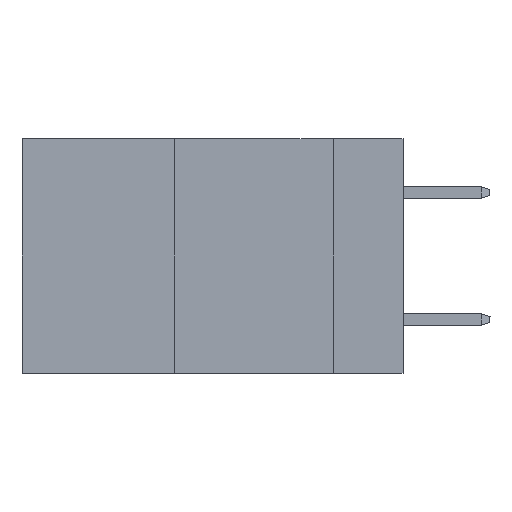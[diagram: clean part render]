
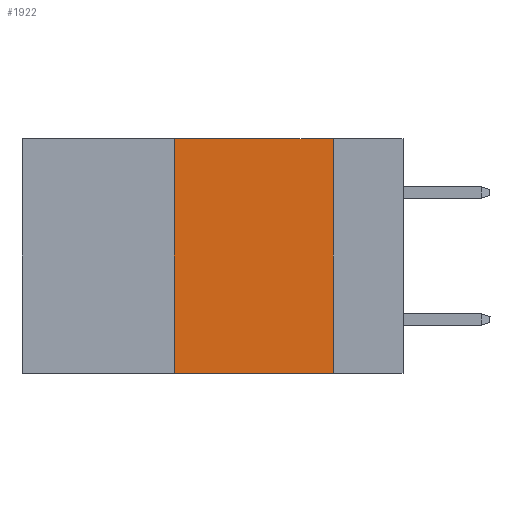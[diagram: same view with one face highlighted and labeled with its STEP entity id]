
A CAD part, left-side view. The second image highlights one B-rep face of the part: STEP entity #1922.
In plain terms, the highlighted planar face has unit normal (-1, 0, 0).
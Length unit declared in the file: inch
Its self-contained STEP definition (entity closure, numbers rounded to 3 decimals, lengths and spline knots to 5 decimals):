
#661 = CARTESIAN_POINT ( 'NONE',  ( 0., 0.11, -0.37 ) ) ;
#853 = ORIENTED_EDGE ( 'NONE', *, *, #22373, .F. ) ;
#1360 = VECTOR ( 'NONE', #24112, 39.37008 ) ;
#1922 = ADVANCED_FACE ( 'NONE', ( #19017 ), #7558, .F. ) ;
#2053 = EDGE_CURVE ( 'NONE', #28522, #11244, #5907, .T. ) ;
#2545 = LINE ( 'NONE', #27266, #9186 ) ;
#3667 = CARTESIAN_POINT ( 'NONE',  ( 0., 0.36, -0.37 ) ) ;
#5485 = LINE ( 'NONE', #28543, #5537 ) ;
#5537 = VECTOR ( 'NONE', #14390, 39.37008 ) ;
#5697 = CARTESIAN_POINT ( 'NONE',  ( 0., 0.6, -0.37 ) ) ;
#5907 = LINE ( 'NONE', #10567, #8036 ) ;
#6410 = VERTEX_POINT ( 'NONE', #3667 ) ;
#6632 = AXIS2_PLACEMENT_3D ( 'NONE', #14051, #23275, #7260 ) ;
#7260 = DIRECTION ( 'NONE',  ( 0., 0., -1. ) ) ;
#7558 = PLANE ( 'NONE',  #6632 ) ;
#8036 = VECTOR ( 'NONE', #24327, 39.37008 ) ;
#8300 = CARTESIAN_POINT ( 'NONE',  ( 0., 0.11, 0. ) ) ;
#9186 = VECTOR ( 'NONE', #13541, 39.37008 ) ;
#10567 = CARTESIAN_POINT ( 'NONE',  ( 0., 0.6, 0. ) ) ;
#11244 = VERTEX_POINT ( 'NONE', #8300 ) ;
#12092 = ORIENTED_EDGE ( 'NONE', *, *, #2053, .F. ) ;
#13541 = DIRECTION ( 'NONE',  ( 0., 0., 1. ) ) ;
#14051 = CARTESIAN_POINT ( 'NONE',  ( 0., 0.6, 0. ) ) ;
#14390 = DIRECTION ( 'NONE',  ( 0., 0., -1. ) ) ;
#16536 = VERTEX_POINT ( 'NONE', #661 ) ;
#18637 = EDGE_CURVE ( 'NONE', #6410, #28522, #2545, .T. ) ;
#19017 = FACE_OUTER_BOUND ( 'NONE', #22444, .T. ) ;
#22242 = ORIENTED_EDGE ( 'NONE', *, *, #18637, .F. ) ;
#22373 = EDGE_CURVE ( 'NONE', #11244, #16536, #5485, .T. ) ;
#22444 = EDGE_LOOP ( 'NONE', ( #853, #12092, #22242, #25065 ) ) ;
#22584 = CARTESIAN_POINT ( 'NONE',  ( 0., 0.36, 0. ) ) ;
#23275 = DIRECTION ( 'NONE',  ( 1., 0., 0. ) ) ;
#24112 = DIRECTION ( 'NONE',  ( 0., -1., 0. ) ) ;
#24327 = DIRECTION ( 'NONE',  ( 0., -1., 0. ) ) ;
#25065 = ORIENTED_EDGE ( 'NONE', *, *, #28432, .T. ) ;
#26342 = LINE ( 'NONE', #5697, #1360 ) ;
#27266 = CARTESIAN_POINT ( 'NONE',  ( 0., 0.36, 0. ) ) ;
#28432 = EDGE_CURVE ( 'NONE', #6410, #16536, #26342, .T. ) ;
#28522 = VERTEX_POINT ( 'NONE', #22584 ) ;
#28543 = CARTESIAN_POINT ( 'NONE',  ( 0., 0.11, 0. ) ) ;
